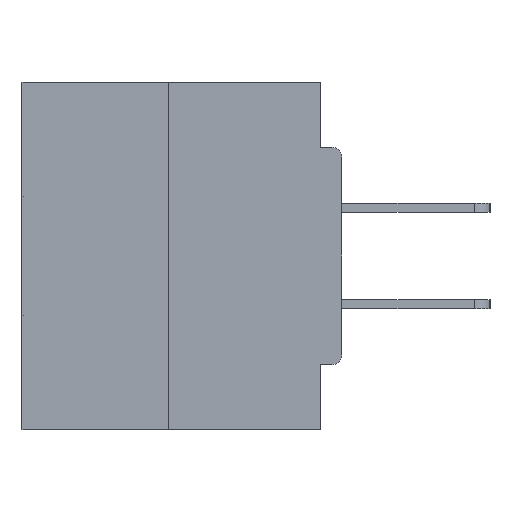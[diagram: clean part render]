
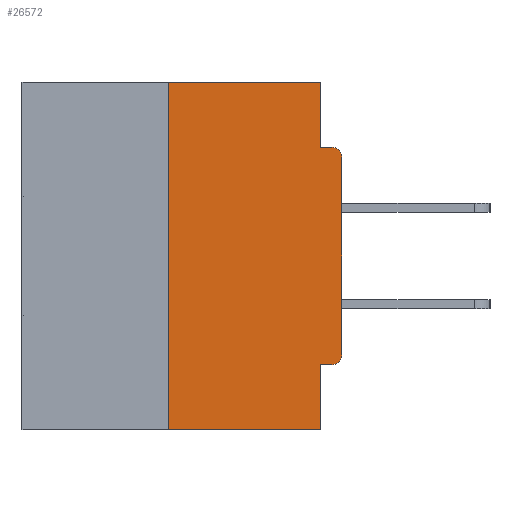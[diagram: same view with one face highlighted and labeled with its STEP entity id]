
A CAD part, left-side view. The second image highlights one B-rep face of the part: STEP entity #26572.
In plain terms, the highlighted planar face has unit normal (-1, 0, 0).
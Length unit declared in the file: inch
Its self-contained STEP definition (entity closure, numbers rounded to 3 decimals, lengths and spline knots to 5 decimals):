
#49 = EDGE_LOOP ( 'NONE', ( #15934, #30597, #2172, #28120, #28768, #14676, #8343, #35333, #17383, #26718 ) ) ;
#895 = DIRECTION ( 'NONE',  ( -1., 0., 0. ) ) ;
#946 = VECTOR ( 'NONE', #12953, 39.37008 ) ;
#1220 = VERTEX_POINT ( 'NONE', #34084 ) ;
#2172 = ORIENTED_EDGE ( 'NONE', *, *, #11573, .T. ) ;
#2473 = CARTESIAN_POINT ( 'NONE',  ( 0., 0.031, -0.5 ) ) ;
#3183 = CARTESIAN_POINT ( 'NONE',  ( 0., 0.031, -0.4065 ) ) ;
#4953 = CARTESIAN_POINT ( 'NONE',  ( 0., 0.031, -0.5 ) ) ;
#4992 = CARTESIAN_POINT ( 'NONE',  ( 0., 0.46, 0. ) ) ;
#6556 = LINE ( 'NONE', #4953, #36858 ) ;
#7207 = CARTESIAN_POINT ( 'NONE',  ( 0., 0., 0. ) ) ;
#8339 = CARTESIAN_POINT ( 'NONE',  ( 0., 0.031, -0.0935 ) ) ;
#8343 = ORIENTED_EDGE ( 'NONE', *, *, #12896, .T. ) ;
#8435 = VECTOR ( 'NONE', #26511, 39.37008 ) ;
#9337 = LINE ( 'NONE', #4992, #33695 ) ;
#10383 = VERTEX_POINT ( 'NONE', #33403 ) ;
#10517 = DIRECTION ( 'NONE',  ( 0., 1., 0. ) ) ;
#11573 = EDGE_CURVE ( 'NONE', #1220, #18674, #19019, .T. ) ;
#11735 = CARTESIAN_POINT ( 'NONE',  ( 0., 0.46, 0. ) ) ;
#11952 = AXIS2_PLACEMENT_3D ( 'NONE', #11735, #32270, #14702 ) ;
#12018 = VERTEX_POINT ( 'NONE', #17464 ) ;
#12593 = EDGE_CURVE ( 'NONE', #20282, #33333, #35017, .T. ) ;
#12896 = EDGE_CURVE ( 'NONE', #23034, #10383, #18912, .T. ) ;
#12953 = DIRECTION ( 'NONE',  ( 0., -1., 0. ) ) ;
#13005 = CARTESIAN_POINT ( 'NONE',  ( 0., 0.015, -0.4065 ) ) ;
#14676 = ORIENTED_EDGE ( 'NONE', *, *, #22986, .T. ) ;
#14702 = DIRECTION ( 'NONE',  ( 0., 0., -1. ) ) ;
#14752 = EDGE_CURVE ( 'NONE', #10383, #15249, #37248, .T. ) ;
#14806 = EDGE_CURVE ( 'NONE', #33042, #15249, #16576, .T. ) ;
#15249 = VERTEX_POINT ( 'NONE', #18089 ) ;
#15830 = EDGE_CURVE ( 'NONE', #12018, #33042, #19704, .T. ) ;
#15919 = CARTESIAN_POINT ( 'NONE',  ( 0., 0.015, -0.1085 ) ) ;
#15934 = ORIENTED_EDGE ( 'NONE', *, *, #25756, .F. ) ;
#16576 = LINE ( 'NONE', #18758, #946 ) ;
#16835 = CARTESIAN_POINT ( 'NONE',  ( 0., 0., -0.4065 ) ) ;
#16954 = VERTEX_POINT ( 'NONE', #21125 ) ;
#17138 = DIRECTION ( 'NONE',  ( 0., 0., 1. ) ) ;
#17266 = CARTESIAN_POINT ( 'NONE',  ( 0., 0.25, 0. ) ) ;
#17383 = ORIENTED_EDGE ( 'NONE', *, *, #14806, .F. ) ;
#17464 = CARTESIAN_POINT ( 'NONE',  ( 0., 0.031, 0. ) ) ;
#17891 = VECTOR ( 'NONE', #35872, 39.37008 ) ;
#18089 = CARTESIAN_POINT ( 'NONE',  ( 0., 0.015, -0.0935 ) ) ;
#18565 = CARTESIAN_POINT ( 'NONE',  ( 0., 0.031, 0. ) ) ;
#18674 = VERTEX_POINT ( 'NONE', #2473 ) ;
#18758 = CARTESIAN_POINT ( 'NONE',  ( 0., 0., -0.0935 ) ) ;
#18912 = LINE ( 'NONE', #7207, #28534 ) ;
#19019 = LINE ( 'NONE', #27530, #8435 ) ;
#19704 = LINE ( 'NONE', #18565, #17891 ) ;
#20101 = DIRECTION ( 'NONE',  ( 0., 0., -1. ) ) ;
#20282 = VERTEX_POINT ( 'NONE', #13005 ) ;
#21125 = CARTESIAN_POINT ( 'NONE',  ( 0., 0.25, 0. ) ) ;
#21557 = DIRECTION ( 'NONE',  ( 0., 0., -1. ) ) ;
#21735 = VECTOR ( 'NONE', #17138, 39.37008 ) ;
#22986 = EDGE_CURVE ( 'NONE', #20282, #23034, #28383, .T. ) ;
#23034 = VERTEX_POINT ( 'NONE', #34035 ) ;
#25524 = DIRECTION ( 'NONE',  ( 0., -1., 0. ) ) ;
#25756 = EDGE_CURVE ( 'NONE', #16954, #12018, #9337, .T. ) ;
#26511 = DIRECTION ( 'NONE',  ( 0., -1., 0. ) ) ;
#26572 = ADVANCED_FACE ( 'NONE', ( #34487 ), #29343, .F. ) ;
#26718 = ORIENTED_EDGE ( 'NONE', *, *, #15830, .F. ) ;
#27530 = CARTESIAN_POINT ( 'NONE',  ( 0., 0.46, -0.5 ) ) ;
#27739 = DIRECTION ( 'NONE',  ( 0., 0., -1. ) ) ;
#27865 = DIRECTION ( 'NONE',  ( -1., 0., 0. ) ) ;
#27986 = DIRECTION ( 'NONE',  ( 0., 0., 1. ) ) ;
#28120 = ORIENTED_EDGE ( 'NONE', *, *, #31791, .F. ) ;
#28383 = CIRCLE ( 'NONE', #29819, 0.015 ) ;
#28534 = VECTOR ( 'NONE', #27986, 39.37008 ) ;
#28768 = ORIENTED_EDGE ( 'NONE', *, *, #12593, .F. ) ;
#29343 = PLANE ( 'NONE',  #11952 ) ;
#29819 = AXIS2_PLACEMENT_3D ( 'NONE', #30807, #27865, #27739 ) ;
#30465 = LINE ( 'NONE', #17266, #21735 ) ;
#30560 = EDGE_CURVE ( 'NONE', #1220, #16954, #30465, .T. ) ;
#30597 = ORIENTED_EDGE ( 'NONE', *, *, #30560, .F. ) ;
#30807 = CARTESIAN_POINT ( 'NONE',  ( 0., 0.015, -0.3915 ) ) ;
#31439 = AXIS2_PLACEMENT_3D ( 'NONE', #15919, #895, #21557 ) ;
#31791 = EDGE_CURVE ( 'NONE', #33333, #18674, #6556, .T. ) ;
#32270 = DIRECTION ( 'NONE',  ( 1., 0., 0. ) ) ;
#33042 = VERTEX_POINT ( 'NONE', #8339 ) ;
#33333 = VERTEX_POINT ( 'NONE', #3183 ) ;
#33403 = CARTESIAN_POINT ( 'NONE',  ( 0., 0., -0.1085 ) ) ;
#33695 = VECTOR ( 'NONE', #25524, 39.37008 ) ;
#34035 = CARTESIAN_POINT ( 'NONE',  ( 0., 0., -0.3915 ) ) ;
#34084 = CARTESIAN_POINT ( 'NONE',  ( 0., 0.25, -0.5 ) ) ;
#34487 = FACE_OUTER_BOUND ( 'NONE', #49, .T. ) ;
#35017 = LINE ( 'NONE', #16835, #36842 ) ;
#35333 = ORIENTED_EDGE ( 'NONE', *, *, #14752, .T. ) ;
#35872 = DIRECTION ( 'NONE',  ( 0., 0., -1. ) ) ;
#36842 = VECTOR ( 'NONE', #10517, 39.37008 ) ;
#36858 = VECTOR ( 'NONE', #20101, 39.37008 ) ;
#37248 = CIRCLE ( 'NONE', #31439, 0.015 ) ;
